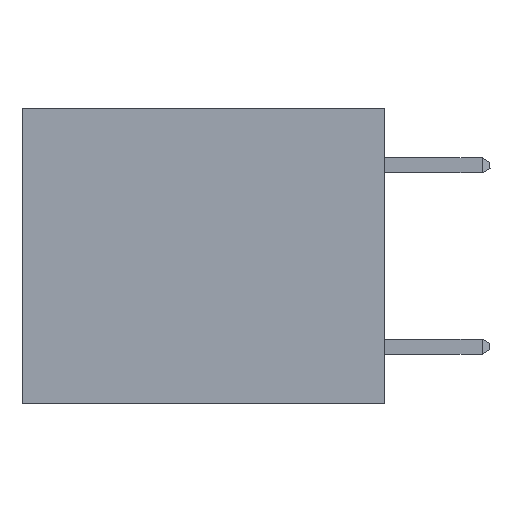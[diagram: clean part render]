
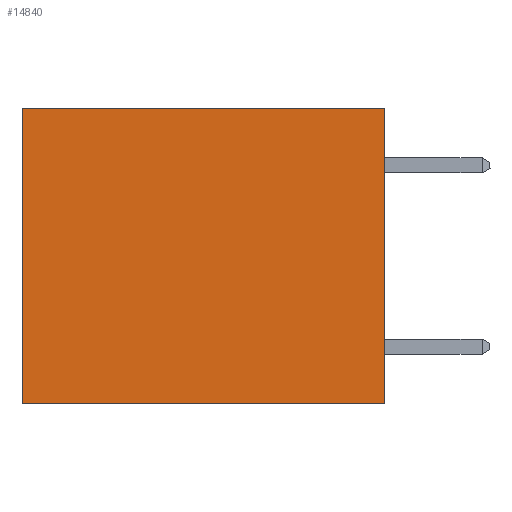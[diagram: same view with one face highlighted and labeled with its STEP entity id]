
A CAD part, left-side view. The second image highlights one B-rep face of the part: STEP entity #14840.
In plain terms, the highlighted planar face has unit normal (-1, 0, 0).
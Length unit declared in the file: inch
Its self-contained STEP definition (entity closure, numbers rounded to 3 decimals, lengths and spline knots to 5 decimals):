
#175 = VERTEX_POINT ( 'NONE', #8732 ) ;
#370 = DIRECTION ( 'NONE',  ( 1., 0., 0. ) ) ;
#2649 = VECTOR ( 'NONE', #8110, 39.37008 ) ;
#3312 = ORIENTED_EDGE ( 'NONE', *, *, #15794, .F. ) ;
#4065 = CARTESIAN_POINT ( 'NONE',  ( 0.3165, 0., 0. ) ) ;
#4346 = VECTOR ( 'NONE', #11556, 39.37008 ) ;
#5011 = VECTOR ( 'NONE', #16946, 39.37008 ) ;
#5152 = EDGE_CURVE ( 'NONE', #20715, #175, #9835, .T. ) ;
#5339 = VERTEX_POINT ( 'NONE', #19859 ) ;
#5642 = EDGE_CURVE ( 'NONE', #12751, #5339, #21246, .T. ) ;
#8110 = DIRECTION ( 'NONE',  ( 0., 0., -1. ) ) ;
#8732 = CARTESIAN_POINT ( 'NONE',  ( 0.3165, 0., -0.49 ) ) ;
#9499 = PLANE ( 'NONE',  #10183 ) ;
#9835 = LINE ( 'NONE', #20824, #2649 ) ;
#9996 = DIRECTION ( 'NONE',  ( 0., 1., 0. ) ) ;
#10183 = AXIS2_PLACEMENT_3D ( 'NONE', #22528, #370, #18690 ) ;
#10649 = ORIENTED_EDGE ( 'NONE', *, *, #5152, .F. ) ;
#11556 = DIRECTION ( 'NONE',  ( 0., 0., -1. ) ) ;
#12257 = ORIENTED_EDGE ( 'NONE', *, *, #15713, .T. ) ;
#12751 = VERTEX_POINT ( 'NONE', #18339 ) ;
#13356 = FACE_OUTER_BOUND ( 'NONE', #15744, .T. ) ;
#14202 = LINE ( 'NONE', #22795, #16179 ) ;
#14840 = ADVANCED_FACE ( 'NONE', ( #13356 ), #9499, .F. ) ;
#15713 = EDGE_CURVE ( 'NONE', #20715, #12751, #16470, .T. ) ;
#15744 = EDGE_LOOP ( 'NONE', ( #20705, #3312, #10649, #12257 ) ) ;
#15794 = EDGE_CURVE ( 'NONE', #175, #5339, #14202, .T. ) ;
#16179 = VECTOR ( 'NONE', #9996, 39.37008 ) ;
#16470 = LINE ( 'NONE', #4065, #5011 ) ;
#16946 = DIRECTION ( 'NONE',  ( 0., 1., 0. ) ) ;
#18339 = CARTESIAN_POINT ( 'NONE',  ( 0.3165, 0.6, 0. ) ) ;
#18690 = DIRECTION ( 'NONE',  ( 0., 0., -1. ) ) ;
#19859 = CARTESIAN_POINT ( 'NONE',  ( 0.3165, 0.6, -0.49 ) ) ;
#20247 = CARTESIAN_POINT ( 'NONE',  ( 0.3165, 0., 0. ) ) ;
#20657 = CARTESIAN_POINT ( 'NONE',  ( 0.3165, 0.6, -0.49 ) ) ;
#20705 = ORIENTED_EDGE ( 'NONE', *, *, #5642, .T. ) ;
#20715 = VERTEX_POINT ( 'NONE', #20247 ) ;
#20824 = CARTESIAN_POINT ( 'NONE',  ( 0.3165, 0., -0.49 ) ) ;
#21246 = LINE ( 'NONE', #20657, #4346 ) ;
#22528 = CARTESIAN_POINT ( 'NONE',  ( 0.3165, 0., -0.49 ) ) ;
#22795 = CARTESIAN_POINT ( 'NONE',  ( 0.3165, 0., -0.49 ) ) ;
